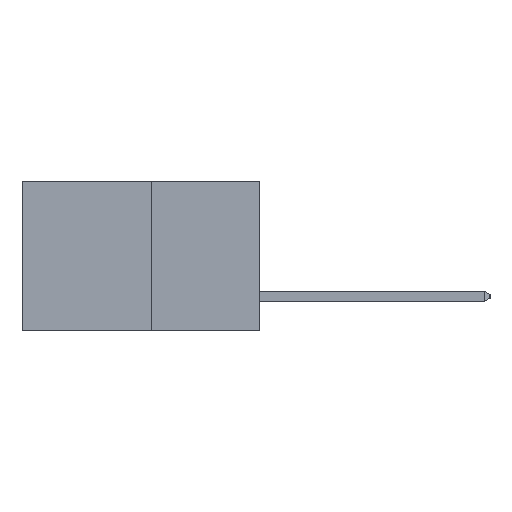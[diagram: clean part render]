
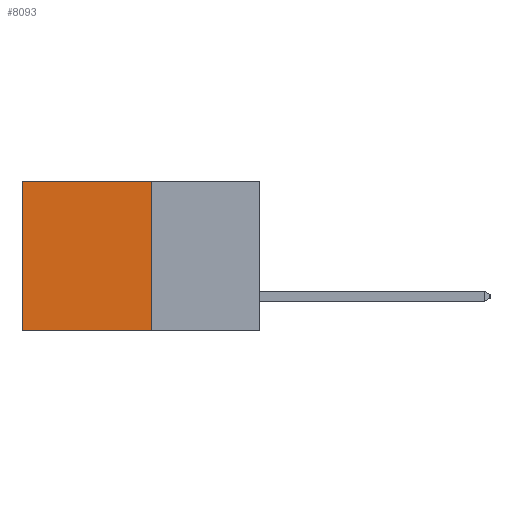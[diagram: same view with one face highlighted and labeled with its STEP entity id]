
A CAD part, left-side view. The second image highlights one B-rep face of the part: STEP entity #8093.
In plain terms, the highlighted planar face has unit normal (-1, 0, 0).
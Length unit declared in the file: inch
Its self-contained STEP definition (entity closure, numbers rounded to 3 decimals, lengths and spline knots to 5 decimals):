
#556 = DIRECTION ( 'NONE',  ( 0., 0., -1. ) ) ;
#601 = DIRECTION ( 'NONE',  ( 1., 0., 0. ) ) ;
#607 = PLANE ( 'NONE',  #823 ) ;
#633 = CARTESIAN_POINT ( 'NONE',  ( 0.277, 0.27, 0. ) ) ;
#795 = CARTESIAN_POINT ( 'NONE',  ( 0.277, 0.27, -0.37 ) ) ;
#802 = EDGE_CURVE ( 'NONE', #7258, #1894, #10528, .T. ) ;
#823 = AXIS2_PLACEMENT_3D ( 'NONE', #795, #601, #556 ) ;
#1686 = DIRECTION ( 'NONE',  ( 0., 1., 0. ) ) ;
#1894 = VERTEX_POINT ( 'NONE', #3712 ) ;
#2250 = VECTOR ( 'NONE', #7637, 39.37008 ) ;
#2507 = VERTEX_POINT ( 'NONE', #3108 ) ;
#3108 = CARTESIAN_POINT ( 'NONE',  ( 0.277, 0.59, 0. ) ) ;
#3459 = ORIENTED_EDGE ( 'NONE', *, *, #4631, .T. ) ;
#3474 = ORIENTED_EDGE ( 'NONE', *, *, #3569, .F. ) ;
#3496 = ORIENTED_EDGE ( 'NONE', *, *, #802, .F. ) ;
#3505 = ORIENTED_EDGE ( 'NONE', *, *, #5905, .T. ) ;
#3569 = EDGE_CURVE ( 'NONE', #1894, #8405, #8356, .T. ) ;
#3712 = CARTESIAN_POINT ( 'NONE',  ( 0.277, 0.27, -0.37 ) ) ;
#4466 = CARTESIAN_POINT ( 'NONE',  ( 0.277, 0.27, -0.37 ) ) ;
#4631 = EDGE_CURVE ( 'NONE', #2507, #8405, #6645, .T. ) ;
#4695 = LINE ( 'NONE', #6718, #2250 ) ;
#5894 = CARTESIAN_POINT ( 'NONE',  ( 0.277, 0.27, -0.37 ) ) ;
#5905 = EDGE_CURVE ( 'NONE', #7258, #2507, #4695, .T. ) ;
#6354 = VECTOR ( 'NONE', #9276, 39.37008 ) ;
#6645 = LINE ( 'NONE', #10666, #10325 ) ;
#6718 = CARTESIAN_POINT ( 'NONE',  ( 0.277, 0.27, 0. ) ) ;
#7258 = VERTEX_POINT ( 'NONE', #633 ) ;
#7637 = DIRECTION ( 'NONE',  ( 0., 1., 0. ) ) ;
#7790 = CARTESIAN_POINT ( 'NONE',  ( 0.277, 0.59, -0.37 ) ) ;
#7836 = VECTOR ( 'NONE', #1686, 39.37008 ) ;
#8093 = ADVANCED_FACE ( 'NONE', ( #8536 ), #607, .F. ) ;
#8356 = LINE ( 'NONE', #5894, #7836 ) ;
#8405 = VERTEX_POINT ( 'NONE', #7790 ) ;
#8536 = FACE_OUTER_BOUND ( 'NONE', #8968, .T. ) ;
#8968 = EDGE_LOOP ( 'NONE', ( #3459, #3474, #3496, #3505 ) ) ;
#9276 = DIRECTION ( 'NONE',  ( 0., 0., -1. ) ) ;
#10325 = VECTOR ( 'NONE', #10747, 39.37008 ) ;
#10528 = LINE ( 'NONE', #4466, #6354 ) ;
#10666 = CARTESIAN_POINT ( 'NONE',  ( 0.277, 0.59, -0.37 ) ) ;
#10747 = DIRECTION ( 'NONE',  ( 0., 0., -1. ) ) ;
